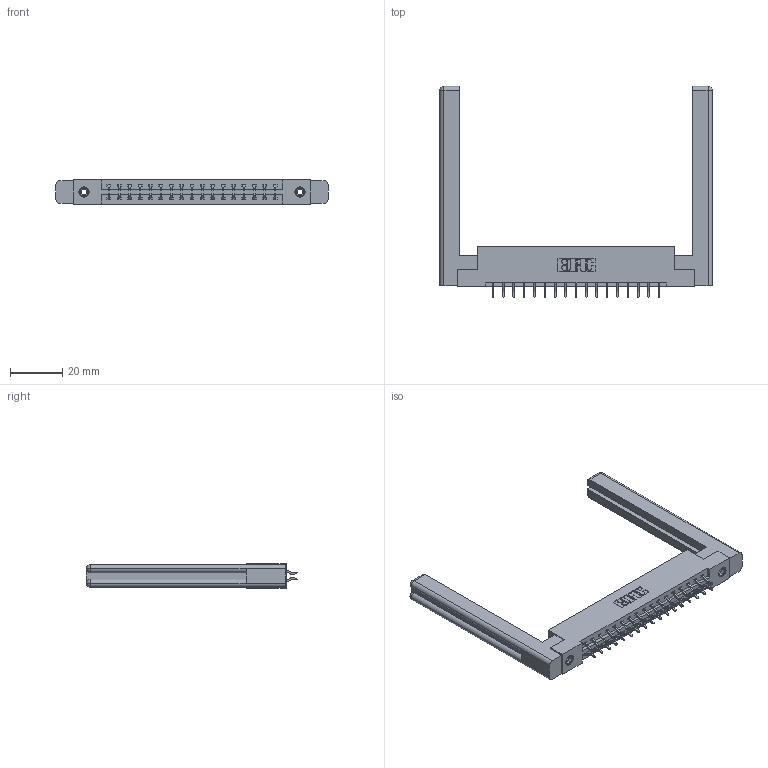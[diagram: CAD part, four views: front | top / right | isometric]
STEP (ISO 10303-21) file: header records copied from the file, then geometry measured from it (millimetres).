
FILE_DESCRIPTION (( 'STEP AP203' ), '1' );
FILE_NAME ('387-034-556-258.STEP', '2019-10-17T18:04:53', ( '' ), ( '' ), 'SwSTEP 2.0', 'SolidWorks 2016', '' );
FILE_SCHEMA (( 'CONFIG_CONTROL_DESIGN' ));
Length unit declared in the file: inch
Products named in the file (5): 387-034-556-258; 307-220-058; 345-250-001_345-250-001-102; 345-292-001_556 Tail; 337 Part_Flush Mounting Lugs - 0.156 Dia-TI
Assembly tree (39 placements, depth 2):
  387-034-556-258
    337 Part_Flush Mounting Lugs - 0.156 Dia-TI
    345-292-001_556 Tail  x34
    345-250-001_345-250-001-102  x2
    307-220-058  x2
Bounding box: 103.99 x 80.66 x 9.4 mm (x, y, z)
Volume: 17767.3 mm3; surface area: 16779.5 mm2
Topology: 39 solids, 39 shells, 2296 faces, 6751 edges, 4442 vertices
Faces by surface type: plane 1582, cylinder 690, cone 12, torus 12
Entity records: 19268 total; most frequent: CARTESIAN_POINT 3289, ORIENTED_EDGE 3152, DIRECTION 2848, EDGE_CURVE 1576, LINE 1392, VECTOR 1392, VERTEX_POINT 1042, AXIS2_PLACEMENT_3D 728
